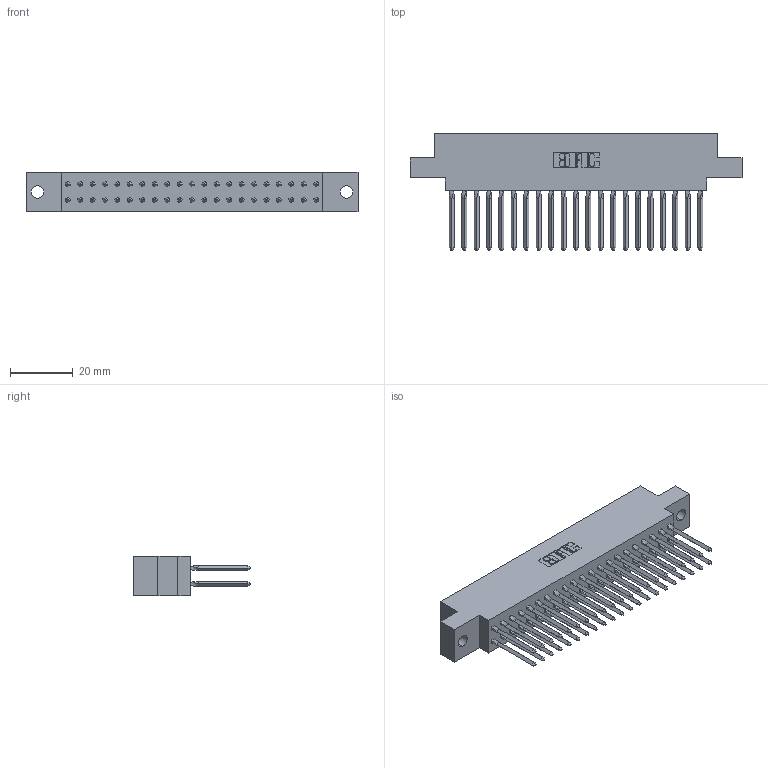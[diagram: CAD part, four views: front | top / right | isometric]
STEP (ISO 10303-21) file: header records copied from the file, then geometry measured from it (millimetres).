
FILE_DESCRIPTION (( 'STEP AP203' ), '1' );
FILE_NAME ('317-042-542-804.STEP', '2020-02-28T01:28:35', ( '' ), ( '' ), 'SwSTEP 2.0', 'SolidWorks 2016', '' );
FILE_SCHEMA (( 'CONFIG_CONTROL_DESIGN' ));
Length unit declared in the file: inch
Products named in the file (3): 317-042-542-804; 317 Part_.156 Dia - TH; 317-290-003_542
Assembly tree (43 placements, depth 2):
  317-042-542-804
    317 Part_.156 Dia - TH
    317-290-003_542  x42
Bounding box: 105.92 x 37.34 x 12.7 mm (x, y, z)
Volume: 16592.2 mm3; surface area: 22216.3 mm2
Topology: 43 solids, 43 shells, 2496 faces, 6995 edges, 4466 vertices
Faces by surface type: plane 1990, cylinder 338, bspline 168
Entity records: 32305 total; most frequent: CARTESIAN_POINT 5881, ORIENTED_EDGE 5544, DIRECTION 4700, EDGE_CURVE 2772, LINE 2602, VECTOR 2602, VERTEX_POINT 1842, AXIS2_PLACEMENT_3D 1049
